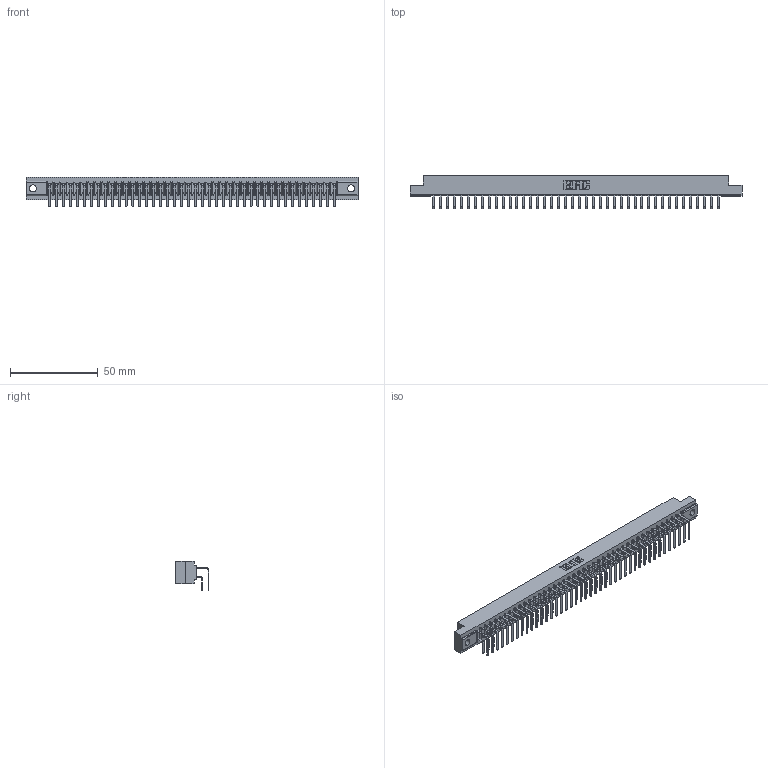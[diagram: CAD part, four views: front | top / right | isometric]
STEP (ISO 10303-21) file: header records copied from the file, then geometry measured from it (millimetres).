
FILE_DESCRIPTION (( 'STEP AP203' ), '1' );
FILE_NAME ('357-084-558-204.STEP', '2018-08-13T01:46:09', ( '' ), ( '' ), 'SwSTEP 2.0', 'SolidWorks 2016', '' );
FILE_SCHEMA (( 'CONFIG_CONTROL_DESIGN' ));
Length unit declared in the file: inch
Products named in the file (4): 357-084-558-204; 307 Part_.156 Dia Mounting Holes; 307-290-001_558 559 - 1 (Single); 307-290-001_558 - 2 (Single)
Assembly tree (85 placements, depth 2):
  357-084-558-204
    307 Part_.156 Dia Mounting Holes
    307-290-001_558 559 - 1 (Single)  x42
    307-290-001_558 - 2 (Single)  x42
Bounding box: 189.43 x 18.96 x 16.8 mm (x, y, z)
Volume: 20410.4 mm3; surface area: 26976.2 mm2
Topology: 85 solids, 85 shells, 4375 faces, 12287 edges, 7962 vertices
Faces by surface type: plane 2856, cylinder 1433, sphere 86
Entity records: 39215 total; most frequent: CARTESIAN_POINT 6422, ORIENTED_EDGE 6362, DIRECTION 6281, EDGE_CURVE 3181, VECTOR 2447, LINE 2447, VERTEX_POINT 2058, AXIS2_PLACEMENT_3D 1917
